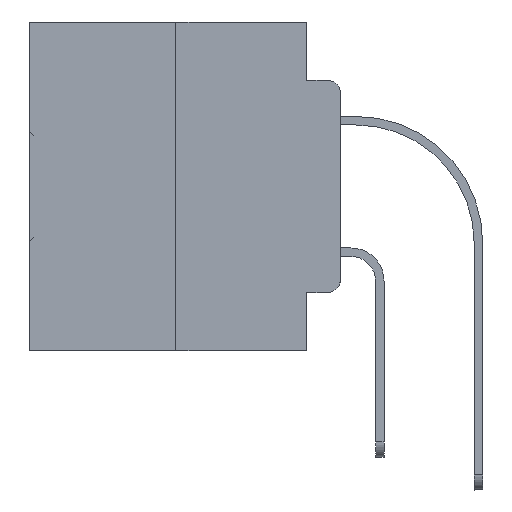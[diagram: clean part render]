
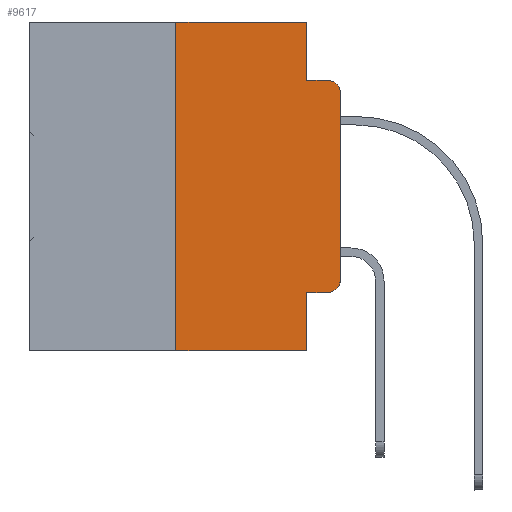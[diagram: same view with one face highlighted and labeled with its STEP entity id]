
A CAD part, left-side view. The second image highlights one B-rep face of the part: STEP entity #9617.
In plain terms, the highlighted planar face has unit normal (-1, 0, 0).
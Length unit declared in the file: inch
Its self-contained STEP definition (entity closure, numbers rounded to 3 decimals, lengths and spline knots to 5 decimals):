
#186 = VERTEX_POINT ( 'NONE', #10093 ) ;
#526 = CARTESIAN_POINT ( 'NONE',  ( 0., 0.473, 0. ) ) ;
#670 = CARTESIAN_POINT ( 'NONE',  ( 0., 0.051, -0.4115 ) ) ;
#794 = CARTESIAN_POINT ( 'NONE',  ( 0., 0.473, 0. ) ) ;
#1492 = ORIENTED_EDGE ( 'NONE', *, *, #4338, .F. ) ;
#1567 = ORIENTED_EDGE ( 'NONE', *, *, #19689, .T. ) ;
#1789 = EDGE_LOOP ( 'NONE', ( #18338, #1567, #19667, #8329, #1492, #9756, #14503, #25505, #34481, #26549 ) ) ;
#3235 = VERTEX_POINT ( 'NONE', #31499 ) ;
#3297 = VECTOR ( 'NONE', #28636, 39.37008 ) ;
#3351 = DIRECTION ( 'NONE',  ( 0., 0., 1. ) ) ;
#3503 = VERTEX_POINT ( 'NONE', #8221 ) ;
#3612 = CARTESIAN_POINT ( 'NONE',  ( 0., 0.02, -0.1085 ) ) ;
#3751 = CARTESIAN_POINT ( 'NONE',  ( 0., 0.473, -0.5 ) ) ;
#3853 = DIRECTION ( 'NONE',  ( 0., 0., -1. ) ) ;
#3884 = DIRECTION ( 'NONE',  ( 0., -1., 0. ) ) ;
#4019 = VECTOR ( 'NONE', #3853, 39.37008 ) ;
#4338 = EDGE_CURVE ( 'NONE', #3235, #7281, #27751, .T. ) ;
#5705 = CIRCLE ( 'NONE', #21673, 0.02 ) ;
#5774 = DIRECTION ( 'NONE',  ( 0., 0., -1. ) ) ;
#6295 = DIRECTION ( 'NONE',  ( -1., 0., 0. ) ) ;
#6536 = FACE_OUTER_BOUND ( 'NONE', #1789, .T. ) ;
#6630 = VECTOR ( 'NONE', #32769, 39.37008 ) ;
#7281 = VERTEX_POINT ( 'NONE', #33484 ) ;
#7307 = EDGE_CURVE ( 'NONE', #14156, #31510, #9640, .T. ) ;
#7783 = CARTESIAN_POINT ( 'NONE',  ( 0., 0., -0.3915 ) ) ;
#7859 = DIRECTION ( 'NONE',  ( 0., 0., -1. ) ) ;
#8221 = CARTESIAN_POINT ( 'NONE',  ( 0., 0.02, -0.0885 ) ) ;
#8329 = ORIENTED_EDGE ( 'NONE', *, *, #17650, .F. ) ;
#8469 = VERTEX_POINT ( 'NONE', #21700 ) ;
#8578 = AXIS2_PLACEMENT_3D ( 'NONE', #794, #22992, #17591 ) ;
#9446 = CARTESIAN_POINT ( 'NONE',  ( 0., 0.25, 0. ) ) ;
#9617 = ADVANCED_FACE ( 'NONE', ( #6536 ), #11540, .F. ) ;
#9640 = LINE ( 'NONE', #3751, #3297 ) ;
#9756 = ORIENTED_EDGE ( 'NONE', *, *, #14307, .F. ) ;
#9838 = VECTOR ( 'NONE', #11599, 39.37008 ) ;
#10093 = CARTESIAN_POINT ( 'NONE',  ( 0., 0.051, -0.4115 ) ) ;
#10166 = VERTEX_POINT ( 'NONE', #24926 ) ;
#11540 = PLANE ( 'NONE',  #8578 ) ;
#11599 = DIRECTION ( 'NONE',  ( 0., -1., 0. ) ) ;
#11933 = CARTESIAN_POINT ( 'NONE',  ( 0., 0.051, -0.0885 ) ) ;
#12144 = VECTOR ( 'NONE', #24893, 39.37008 ) ;
#13840 = VECTOR ( 'NONE', #3884, 39.37008 ) ;
#14156 = VERTEX_POINT ( 'NONE', #16248 ) ;
#14265 = LINE ( 'NONE', #670, #9838 ) ;
#14307 = EDGE_CURVE ( 'NONE', #14156, #3235, #30554, .T. ) ;
#14357 = EDGE_CURVE ( 'NONE', #186, #10166, #14265, .T. ) ;
#14447 = EDGE_CURVE ( 'NONE', #33060, #3503, #17310, .T. ) ;
#14503 = ORIENTED_EDGE ( 'NONE', *, *, #7307, .T. ) ;
#16248 = CARTESIAN_POINT ( 'NONE',  ( 0., 0.25, -0.5 ) ) ;
#16621 = AXIS2_PLACEMENT_3D ( 'NONE', #3612, #6295, #5774 ) ;
#16735 = DIRECTION ( 'NONE',  ( 0., 0., -1. ) ) ;
#16940 = EDGE_CURVE ( 'NONE', #10166, #24633, #5705, .T. ) ;
#17003 = CARTESIAN_POINT ( 'NONE',  ( 0., 0.051, -0.5 ) ) ;
#17157 = VECTOR ( 'NONE', #16735, 39.37008 ) ;
#17310 = LINE ( 'NONE', #11933, #13840 ) ;
#17591 = DIRECTION ( 'NONE',  ( 0., 0., -1. ) ) ;
#17650 = EDGE_CURVE ( 'NONE', #7281, #33060, #30356, .T. ) ;
#17827 = VECTOR ( 'NONE', #3351, 39.37008 ) ;
#18338 = ORIENTED_EDGE ( 'NONE', *, *, #29288, .T. ) ;
#19078 = LINE ( 'NONE', #33227, #17157 ) ;
#19667 = ORIENTED_EDGE ( 'NONE', *, *, #14447, .F. ) ;
#19689 = EDGE_CURVE ( 'NONE', #8469, #3503, #28050, .T. ) ;
#21628 = CARTESIAN_POINT ( 'NONE',  ( 0., 0.02, -0.3915 ) ) ;
#21673 = AXIS2_PLACEMENT_3D ( 'NONE', #21628, #24329, #7859 ) ;
#21700 = CARTESIAN_POINT ( 'NONE',  ( 0., 0., -0.1085 ) ) ;
#22992 = DIRECTION ( 'NONE',  ( 1., 0., 0. ) ) ;
#23508 = EDGE_CURVE ( 'NONE', #186, #31510, #19078, .T. ) ;
#24329 = DIRECTION ( 'NONE',  ( -1., 0., 0. ) ) ;
#24633 = VERTEX_POINT ( 'NONE', #7783 ) ;
#24870 = CARTESIAN_POINT ( 'NONE',  ( 0., 0., 0. ) ) ;
#24893 = DIRECTION ( 'NONE',  ( 0., -1., 0. ) ) ;
#24926 = CARTESIAN_POINT ( 'NONE',  ( 0., 0.02, -0.4115 ) ) ;
#25505 = ORIENTED_EDGE ( 'NONE', *, *, #23508, .F. ) ;
#26549 = ORIENTED_EDGE ( 'NONE', *, *, #16940, .T. ) ;
#27751 = LINE ( 'NONE', #526, #12144 ) ;
#28025 = CARTESIAN_POINT ( 'NONE',  ( 0., 0.051, 0. ) ) ;
#28050 = CIRCLE ( 'NONE', #16621, 0.02 ) ;
#28344 = CARTESIAN_POINT ( 'NONE',  ( 0., 0.051, -0.0885 ) ) ;
#28636 = DIRECTION ( 'NONE',  ( 0., -1., 0. ) ) ;
#29288 = EDGE_CURVE ( 'NONE', #24633, #8469, #35272, .T. ) ;
#30356 = LINE ( 'NONE', #28025, #4019 ) ;
#30554 = LINE ( 'NONE', #9446, #17827 ) ;
#31499 = CARTESIAN_POINT ( 'NONE',  ( 0., 0.25, 0. ) ) ;
#31510 = VERTEX_POINT ( 'NONE', #17003 ) ;
#32769 = DIRECTION ( 'NONE',  ( 0., 0., 1. ) ) ;
#33060 = VERTEX_POINT ( 'NONE', #28344 ) ;
#33227 = CARTESIAN_POINT ( 'NONE',  ( 0., 0.051, 0. ) ) ;
#33484 = CARTESIAN_POINT ( 'NONE',  ( 0., 0.051, 0. ) ) ;
#34481 = ORIENTED_EDGE ( 'NONE', *, *, #14357, .T. ) ;
#35272 = LINE ( 'NONE', #24870, #6630 ) ;
